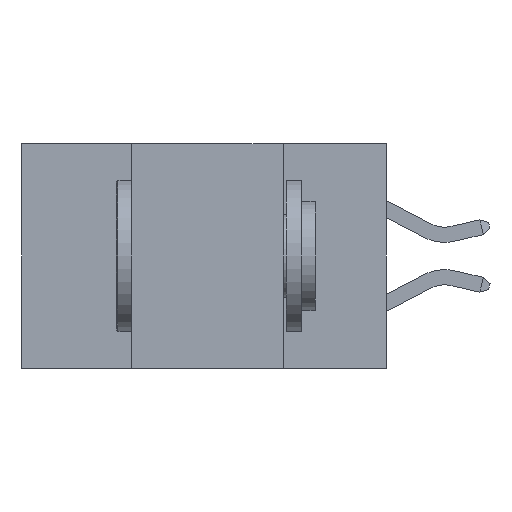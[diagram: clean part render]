
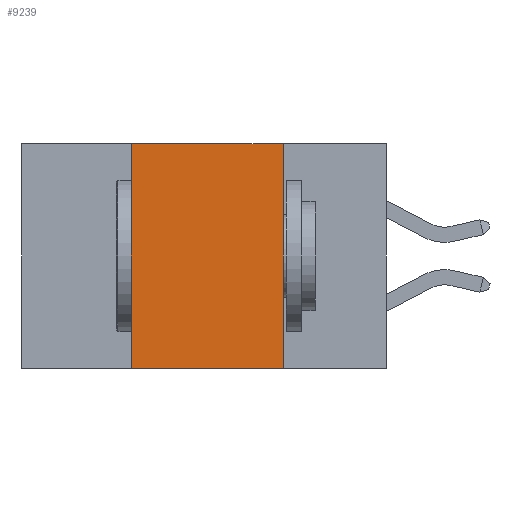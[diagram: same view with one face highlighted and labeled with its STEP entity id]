
A CAD part, left-side view. The second image highlights one B-rep face of the part: STEP entity #9239.
In plain terms, the highlighted planar face has unit normal (-1, 0, 0).
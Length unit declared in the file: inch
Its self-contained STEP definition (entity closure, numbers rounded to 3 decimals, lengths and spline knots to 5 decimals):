
#319 = FACE_OUTER_BOUND ( 'NONE', #16673, .T. ) ;
#964 = ORIENTED_EDGE ( 'NONE', *, *, #5082, .F. ) ;
#1256 = ORIENTED_EDGE ( 'NONE', *, *, #22204, .T. ) ;
#1511 = DIRECTION ( 'NONE',  ( 0., 0., -1. ) ) ;
#1650 = VERTEX_POINT ( 'NONE', #5252 ) ;
#2590 = PLANE ( 'NONE',  #16669 ) ;
#2791 = CARTESIAN_POINT ( 'NONE',  ( 0., 0.42, 0. ) ) ;
#2803 = LINE ( 'NONE', #2791, #10352 ) ;
#3332 = LINE ( 'NONE', #14427, #22472 ) ;
#3407 = DIRECTION ( 'NONE',  ( 0., -1., 0. ) ) ;
#4502 = DIRECTION ( 'NONE',  ( 1., 0., 0. ) ) ;
#5082 = EDGE_CURVE ( 'NONE', #12542, #7031, #10106, .T. ) ;
#5252 = CARTESIAN_POINT ( 'NONE',  ( 0., 0.42, 0. ) ) ;
#5451 = DIRECTION ( 'NONE',  ( 0., 0., -1. ) ) ;
#5827 = VERTEX_POINT ( 'NONE', #19290 ) ;
#7031 = VERTEX_POINT ( 'NONE', #17935 ) ;
#7504 = DIRECTION ( 'NONE',  ( 0., -1., 0. ) ) ;
#9239 = ADVANCED_FACE ( 'NONE', ( #319 ), #2590, .F. ) ;
#10106 = LINE ( 'NONE', #14440, #13286 ) ;
#10156 = LINE ( 'NONE', #16923, #11587 ) ;
#10352 = VECTOR ( 'NONE', #15592, 39.37008 ) ;
#11587 = VECTOR ( 'NONE', #7504, 39.37008 ) ;
#12542 = VERTEX_POINT ( 'NONE', #13330 ) ;
#13286 = VECTOR ( 'NONE', #1511, 39.37008 ) ;
#13330 = CARTESIAN_POINT ( 'NONE',  ( 0., 0.17, 0. ) ) ;
#14427 = CARTESIAN_POINT ( 'NONE',  ( 0., 0.6, -0.37 ) ) ;
#14440 = CARTESIAN_POINT ( 'NONE',  ( 0., 0.17, 0. ) ) ;
#14936 = EDGE_CURVE ( 'NONE', #5827, #1650, #2803, .T. ) ;
#15592 = DIRECTION ( 'NONE',  ( 0., 0., 1. ) ) ;
#16669 = AXIS2_PLACEMENT_3D ( 'NONE', #17410, #4502, #5451 ) ;
#16673 = EDGE_LOOP ( 'NONE', ( #964, #16885, #18811, #1256 ) ) ;
#16885 = ORIENTED_EDGE ( 'NONE', *, *, #19586, .F. ) ;
#16923 = CARTESIAN_POINT ( 'NONE',  ( 0., 0.6, 0. ) ) ;
#17410 = CARTESIAN_POINT ( 'NONE',  ( 0., 0.6, 0. ) ) ;
#17935 = CARTESIAN_POINT ( 'NONE',  ( 0., 0.17, -0.37 ) ) ;
#18811 = ORIENTED_EDGE ( 'NONE', *, *, #14936, .F. ) ;
#19290 = CARTESIAN_POINT ( 'NONE',  ( 0., 0.42, -0.37 ) ) ;
#19586 = EDGE_CURVE ( 'NONE', #1650, #12542, #10156, .T. ) ;
#22204 = EDGE_CURVE ( 'NONE', #5827, #7031, #3332, .T. ) ;
#22472 = VECTOR ( 'NONE', #3407, 39.37008 ) ;
